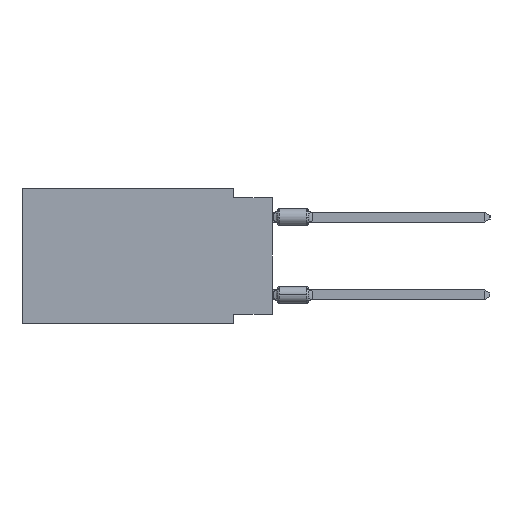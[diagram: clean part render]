
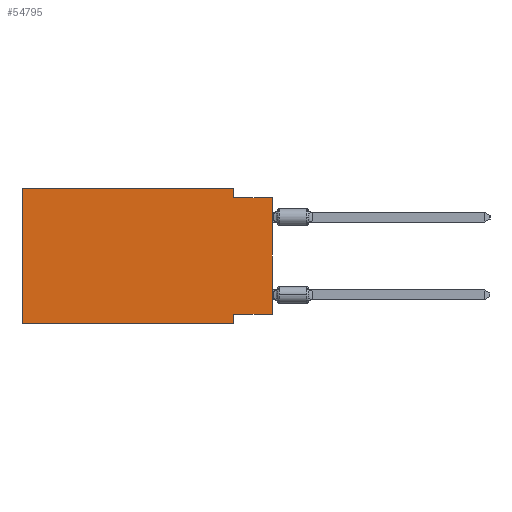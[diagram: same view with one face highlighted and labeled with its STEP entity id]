
A CAD part, left-side view. The second image highlights one B-rep face of the part: STEP entity #54795.
In plain terms, the highlighted planar face has unit normal (-1, 0, 0).
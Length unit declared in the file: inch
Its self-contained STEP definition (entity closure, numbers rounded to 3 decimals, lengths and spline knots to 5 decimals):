
#1113 = CARTESIAN_POINT ( 'NONE',  ( 0., 0.645, -0.35 ) ) ;
#1354 = AXIS2_PLACEMENT_3D ( 'NONE', #4887, #5218, #10835 ) ;
#1572 = DIRECTION ( 'NONE',  ( 0., 0., 1. ) ) ;
#2398 = CARTESIAN_POINT ( 'NONE',  ( 0., 0., -0.025 ) ) ;
#4887 = CARTESIAN_POINT ( 'NONE',  ( 0., 0.645, 0. ) ) ;
#5218 = DIRECTION ( 'NONE',  ( 1., 0., 0. ) ) ;
#5603 = VERTEX_POINT ( 'NONE', #2398 ) ;
#5916 = DIRECTION ( 'NONE',  ( 0., -1., 0. ) ) ;
#7199 = VERTEX_POINT ( 'NONE', #63278 ) ;
#7751 = CARTESIAN_POINT ( 'NONE',  ( 0., 0.1, -0.35 ) ) ;
#8894 = ORIENTED_EDGE ( 'NONE', *, *, #10679, .T. ) ;
#9467 = CARTESIAN_POINT ( 'NONE',  ( 0., 0.645, 0. ) ) ;
#10679 = EDGE_CURVE ( 'NONE', #7199, #5603, #29411, .T. ) ;
#10835 = DIRECTION ( 'NONE',  ( 0., 0., -1. ) ) ;
#11447 = LINE ( 'NONE', #45781, #60726 ) ;
#12856 = VECTOR ( 'NONE', #34743, 39.37008 ) ;
#14180 = CARTESIAN_POINT ( 'NONE',  ( 0., 0.1, -0.325 ) ) ;
#14411 = CARTESIAN_POINT ( 'NONE',  ( 0., 0., 0. ) ) ;
#15839 = PLANE ( 'NONE',  #1354 ) ;
#17390 = EDGE_LOOP ( 'NONE', ( #8894, #43929, #30555, #50174, #54891, #56926, #20536, #27792 ) ) ;
#18350 = DIRECTION ( 'NONE',  ( 0., 0., -1. ) ) ;
#20219 = CARTESIAN_POINT ( 'NONE',  ( 0., 0., -0.025 ) ) ;
#20464 = DIRECTION ( 'NONE',  ( 0., 1., 0. ) ) ;
#20536 = ORIENTED_EDGE ( 'NONE', *, *, #63881, .F. ) ;
#23916 = VECTOR ( 'NONE', #1572, 39.37008 ) ;
#24479 = DIRECTION ( 'NONE',  ( 0., -1., 0. ) ) ;
#26170 = FACE_OUTER_BOUND ( 'NONE', #17390, .T. ) ;
#27078 = DIRECTION ( 'NONE',  ( 0., -1., 0. ) ) ;
#27792 = ORIENTED_EDGE ( 'NONE', *, *, #40765, .F. ) ;
#29411 = LINE ( 'NONE', #14411, #12856 ) ;
#30555 = ORIENTED_EDGE ( 'NONE', *, *, #60191, .F. ) ;
#32854 = LINE ( 'NONE', #63424, #23916 ) ;
#34743 = DIRECTION ( 'NONE',  ( 0., 0., 1. ) ) ;
#36116 = EDGE_CURVE ( 'NONE', #37009, #5603, #46516, .T. ) ;
#37009 = VERTEX_POINT ( 'NONE', #42589 ) ;
#37534 = CARTESIAN_POINT ( 'NONE',  ( 0., 0.1, 0. ) ) ;
#37611 = VERTEX_POINT ( 'NONE', #14180 ) ;
#40627 = EDGE_CURVE ( 'NONE', #53724, #56160, #45440, .T. ) ;
#40765 = EDGE_CURVE ( 'NONE', #7199, #37611, #11447, .T. ) ;
#42589 = CARTESIAN_POINT ( 'NONE',  ( 0., 0.1, -0.025 ) ) ;
#43263 = VERTEX_POINT ( 'NONE', #7751 ) ;
#43666 = CARTESIAN_POINT ( 'NONE',  ( 0., 0.1, -0.35 ) ) ;
#43929 = ORIENTED_EDGE ( 'NONE', *, *, #36116, .F. ) ;
#44012 = VECTOR ( 'NONE', #63093, 39.37008 ) ;
#45440 = LINE ( 'NONE', #54444, #58545 ) ;
#45781 = CARTESIAN_POINT ( 'NONE',  ( 0., 0., -0.325 ) ) ;
#46516 = LINE ( 'NONE', #20219, #62449 ) ;
#46704 = LINE ( 'NONE', #1113, #57548 ) ;
#50174 = ORIENTED_EDGE ( 'NONE', *, *, #40627, .F. ) ;
#50746 = VERTEX_POINT ( 'NONE', #53346 ) ;
#53346 = CARTESIAN_POINT ( 'NONE',  ( 0., 0.645, -0.35 ) ) ;
#53724 = VERTEX_POINT ( 'NONE', #9467 ) ;
#54444 = CARTESIAN_POINT ( 'NONE',  ( 0., 0.645, 0. ) ) ;
#54795 = ADVANCED_FACE ( 'NONE', ( #26170 ), #15839, .F. ) ;
#54891 = ORIENTED_EDGE ( 'NONE', *, *, #61303, .F. ) ;
#56160 = VERTEX_POINT ( 'NONE', #37534 ) ;
#56926 = ORIENTED_EDGE ( 'NONE', *, *, #56956, .T. ) ;
#56956 = EDGE_CURVE ( 'NONE', #50746, #43263, #46704, .T. ) ;
#57548 = VECTOR ( 'NONE', #27078, 39.37008 ) ;
#58545 = VECTOR ( 'NONE', #24479, 39.37008 ) ;
#60191 = EDGE_CURVE ( 'NONE', #56160, #37009, #63413, .T. ) ;
#60726 = VECTOR ( 'NONE', #20464, 39.37008 ) ;
#61261 = VECTOR ( 'NONE', #18350, 39.37008 ) ;
#61303 = EDGE_CURVE ( 'NONE', #50746, #53724, #32854, .T. ) ;
#62449 = VECTOR ( 'NONE', #5916, 39.37008 ) ;
#62759 = CARTESIAN_POINT ( 'NONE',  ( 0., 0.1, 0. ) ) ;
#63093 = DIRECTION ( 'NONE',  ( 0., 0., -1. ) ) ;
#63278 = CARTESIAN_POINT ( 'NONE',  ( 0., 0., -0.325 ) ) ;
#63413 = LINE ( 'NONE', #62759, #44012 ) ;
#63424 = CARTESIAN_POINT ( 'NONE',  ( 0., 0.645, 0. ) ) ;
#63881 = EDGE_CURVE ( 'NONE', #37611, #43263, #64937, .T. ) ;
#64937 = LINE ( 'NONE', #43666, #61261 ) ;
